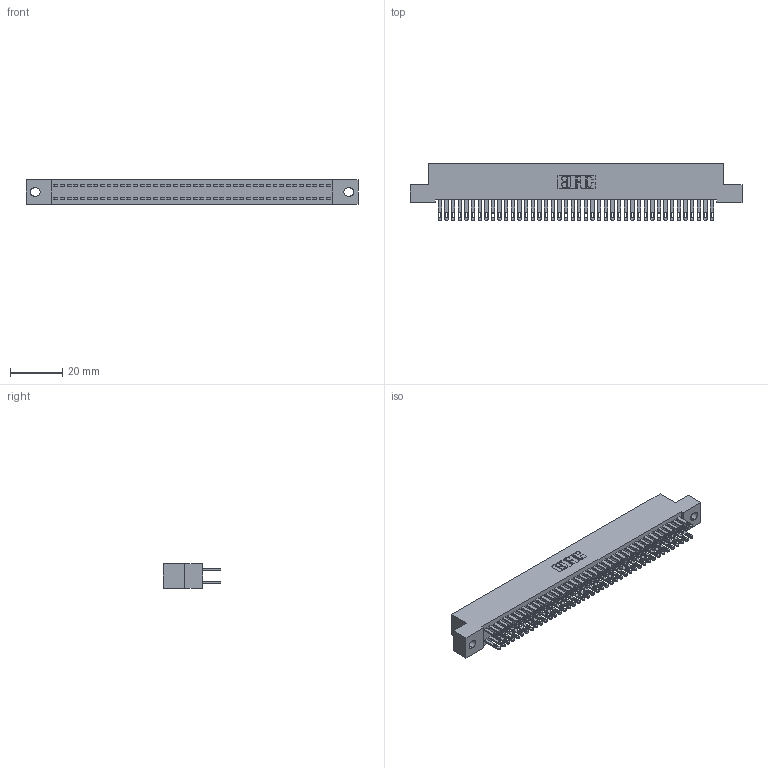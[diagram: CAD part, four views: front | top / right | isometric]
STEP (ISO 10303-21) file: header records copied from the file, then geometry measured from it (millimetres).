
FILE_DESCRIPTION (( 'STEP AP203' ), '1' );
FILE_NAME ('342-084-500-202.STEP', '2018-08-13T17:12:22', ( '' ), ( '' ), 'SwSTEP 2.0', 'SolidWorks 2016', '' );
FILE_SCHEMA (( 'CONFIG_CONTROL_DESIGN' ));
Length unit declared in the file: inch
Products named in the file (3): 342 Part_.128 Slot; 345-292-001_345-293-100; 342-084-500-202
Assembly tree (85 placements, depth 2):
  342-084-500-202
    342 Part_.128 Slot
    345-292-001_345-293-100  x84
Bounding box: 127 x 21.85 x 9.4 mm (x, y, z)
Volume: 11615.5 mm3; surface area: 19470.8 mm2
Topology: 85 solids, 85 shells, 4146 faces, 12659 edges, 8438 vertices
Faces by surface type: plane 2590, cylinder 1556
Entity records: 26953 total; most frequent: CARTESIAN_POINT 4466, ORIENTED_EDGE 4402, DIRECTION 3817, EDGE_CURVE 2201, VECTOR 2069, LINE 2069, VERTEX_POINT 1466, AXIS2_PLACEMENT_3D 874
